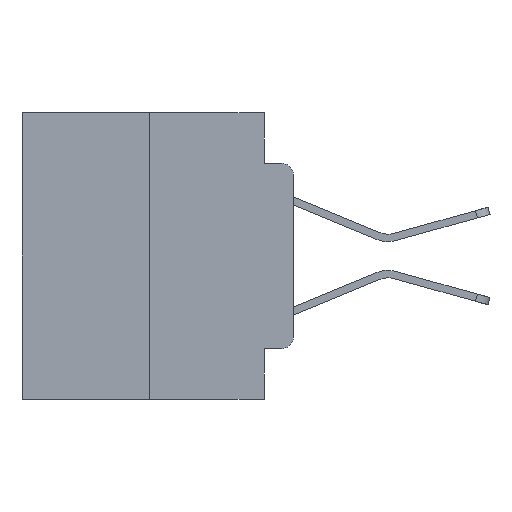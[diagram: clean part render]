
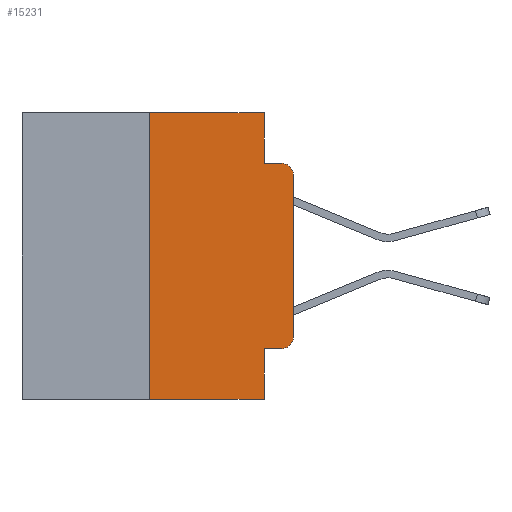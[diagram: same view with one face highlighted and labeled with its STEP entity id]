
A CAD part, left-side view. The second image highlights one B-rep face of the part: STEP entity #15231.
In plain terms, the highlighted planar face has unit normal (-1, 0, 0).
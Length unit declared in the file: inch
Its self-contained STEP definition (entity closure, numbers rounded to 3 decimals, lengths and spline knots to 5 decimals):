
#1120 = VERTEX_POINT ( 'NONE', #7010 ) ;
#1561 = EDGE_CURVE ( 'NONE', #12364, #4137, #19903, .T. ) ;
#2242 = LINE ( 'NONE', #12837, #7956 ) ;
#2682 = ORIENTED_EDGE ( 'NONE', *, *, #17629, .T. ) ;
#2771 = CIRCLE ( 'NONE', #26360, 0.02 ) ;
#3016 = VECTOR ( 'NONE', #15825, 39.37008 ) ;
#3034 = EDGE_CURVE ( 'NONE', #20661, #12364, #10849, .T. ) ;
#3734 = CARTESIAN_POINT ( 'NONE',  ( 0., 0.25, 0. ) ) ;
#4137 = VERTEX_POINT ( 'NONE', #20145 ) ;
#4380 = ORIENTED_EDGE ( 'NONE', *, *, #15844, .T. ) ;
#6556 = CARTESIAN_POINT ( 'NONE',  ( 0., 0.02, -0.3915 ) ) ;
#6719 = CARTESIAN_POINT ( 'NONE',  ( 0., 0.051, -0.5 ) ) ;
#7010 = CARTESIAN_POINT ( 'NONE',  ( 0., 0.051, 0. ) ) ;
#7021 = CARTESIAN_POINT ( 'NONE',  ( 0., 0.051, -0.0885 ) ) ;
#7090 = VERTEX_POINT ( 'NONE', #21341 ) ;
#7255 = CARTESIAN_POINT ( 'NONE',  ( 0., 0.25, 0. ) ) ;
#7353 = EDGE_CURVE ( 'NONE', #20661, #8092, #24828, .T. ) ;
#7412 = VECTOR ( 'NONE', #15946, 39.37008 ) ;
#7582 = DIRECTION ( 'NONE',  ( 0., 0., -1. ) ) ;
#7715 = ORIENTED_EDGE ( 'NONE', *, *, #10358, .F. ) ;
#7956 = VECTOR ( 'NONE', #25434, 39.37008 ) ;
#8092 = VERTEX_POINT ( 'NONE', #6719 ) ;
#8691 = DIRECTION ( 'NONE',  ( -1., 0., 0. ) ) ;
#8750 = EDGE_CURVE ( 'NONE', #7090, #11985, #10701, .T. ) ;
#9026 = ORIENTED_EDGE ( 'NONE', *, *, #7353, .F. ) ;
#9848 = VECTOR ( 'NONE', #23888, 39.37008 ) ;
#10161 = EDGE_CURVE ( 'NONE', #1120, #20254, #20555, .T. ) ;
#10290 = LINE ( 'NONE', #12591, #25115 ) ;
#10358 = EDGE_CURVE ( 'NONE', #11985, #1120, #10290, .T. ) ;
#10461 = DIRECTION ( 'NONE',  ( 0., -1., 0. ) ) ;
#10701 = LINE ( 'NONE', #7255, #16358 ) ;
#10849 = LINE ( 'NONE', #20839, #15846 ) ;
#11060 = EDGE_LOOP ( 'NONE', ( #4380, #15633, #21891, #16959, #7715, #24508, #2682, #9026, #14640, #15301 ) ) ;
#11370 = DIRECTION ( 'NONE',  ( 0., 0., 1. ) ) ;
#11985 = VERTEX_POINT ( 'NONE', #3734 ) ;
#12364 = VERTEX_POINT ( 'NONE', #23922 ) ;
#12434 = DIRECTION ( 'NONE',  ( 0., -1., 0. ) ) ;
#12591 = CARTESIAN_POINT ( 'NONE',  ( 0., 0.473, 0. ) ) ;
#12837 = CARTESIAN_POINT ( 'NONE',  ( 0., 0.473, -0.5 ) ) ;
#12991 = EDGE_CURVE ( 'NONE', #20254, #19797, #26641, .T. ) ;
#13797 = CARTESIAN_POINT ( 'NONE',  ( 0., 0.051, 0. ) ) ;
#14425 = EDGE_CURVE ( 'NONE', #14465, #19797, #2771, .T. ) ;
#14465 = VERTEX_POINT ( 'NONE', #19303 ) ;
#14640 = ORIENTED_EDGE ( 'NONE', *, *, #3034, .T. ) ;
#15209 = CARTESIAN_POINT ( 'NONE',  ( 0., 0.02, -0.0885 ) ) ;
#15231 = ADVANCED_FACE ( 'NONE', ( #17027 ), #15975, .F. ) ;
#15301 = ORIENTED_EDGE ( 'NONE', *, *, #1561, .T. ) ;
#15633 = ORIENTED_EDGE ( 'NONE', *, *, #14425, .T. ) ;
#15747 = CARTESIAN_POINT ( 'NONE',  ( 0., 0.051, -0.4115 ) ) ;
#15825 = DIRECTION ( 'NONE',  ( 0., 0., -1. ) ) ;
#15844 = EDGE_CURVE ( 'NONE', #4137, #14465, #18621, .T. ) ;
#15846 = VECTOR ( 'NONE', #12434, 39.37008 ) ;
#15946 = DIRECTION ( 'NONE',  ( 0., 0., 1. ) ) ;
#15975 = PLANE ( 'NONE',  #17770 ) ;
#16358 = VECTOR ( 'NONE', #11370, 39.37008 ) ;
#16959 = ORIENTED_EDGE ( 'NONE', *, *, #10161, .F. ) ;
#17027 = FACE_OUTER_BOUND ( 'NONE', #11060, .T. ) ;
#17629 = EDGE_CURVE ( 'NONE', #7090, #8092, #2242, .T. ) ;
#17770 = AXIS2_PLACEMENT_3D ( 'NONE', #18090, #20208, #7582 ) ;
#18090 = CARTESIAN_POINT ( 'NONE',  ( 0., 0.473, 0. ) ) ;
#18243 = DIRECTION ( 'NONE',  ( 0., 0., -1. ) ) ;
#18621 = LINE ( 'NONE', #26392, #7412 ) ;
#19303 = CARTESIAN_POINT ( 'NONE',  ( 0., 0., -0.1085 ) ) ;
#19797 = VERTEX_POINT ( 'NONE', #15209 ) ;
#19884 = VECTOR ( 'NONE', #18243, 39.37008 ) ;
#19903 = CIRCLE ( 'NONE', #21220, 0.02 ) ;
#20145 = CARTESIAN_POINT ( 'NONE',  ( 0., 0., -0.3915 ) ) ;
#20208 = DIRECTION ( 'NONE',  ( 1., 0., 0. ) ) ;
#20254 = VERTEX_POINT ( 'NONE', #20813 ) ;
#20448 = DIRECTION ( 'NONE',  ( -1., 0., 0. ) ) ;
#20555 = LINE ( 'NONE', #26575, #19884 ) ;
#20659 = DIRECTION ( 'NONE',  ( 0., 0., -1. ) ) ;
#20661 = VERTEX_POINT ( 'NONE', #15747 ) ;
#20813 = CARTESIAN_POINT ( 'NONE',  ( 0., 0.051, -0.0885 ) ) ;
#20839 = CARTESIAN_POINT ( 'NONE',  ( 0., 0.051, -0.4115 ) ) ;
#21220 = AXIS2_PLACEMENT_3D ( 'NONE', #6556, #20448, #20659 ) ;
#21336 = CARTESIAN_POINT ( 'NONE',  ( 0., 0.02, -0.1085 ) ) ;
#21341 = CARTESIAN_POINT ( 'NONE',  ( 0., 0.25, -0.5 ) ) ;
#21891 = ORIENTED_EDGE ( 'NONE', *, *, #12991, .F. ) ;
#23451 = DIRECTION ( 'NONE',  ( 0., 0., -1. ) ) ;
#23888 = DIRECTION ( 'NONE',  ( 0., -1., 0. ) ) ;
#23922 = CARTESIAN_POINT ( 'NONE',  ( 0., 0.02, -0.4115 ) ) ;
#24508 = ORIENTED_EDGE ( 'NONE', *, *, #8750, .F. ) ;
#24828 = LINE ( 'NONE', #13797, #3016 ) ;
#25115 = VECTOR ( 'NONE', #10461, 39.37008 ) ;
#25434 = DIRECTION ( 'NONE',  ( 0., -1., 0. ) ) ;
#26360 = AXIS2_PLACEMENT_3D ( 'NONE', #21336, #8691, #23451 ) ;
#26392 = CARTESIAN_POINT ( 'NONE',  ( 0., 0., 0. ) ) ;
#26575 = CARTESIAN_POINT ( 'NONE',  ( 0., 0.051, 0. ) ) ;
#26641 = LINE ( 'NONE', #7021, #9848 ) ;
